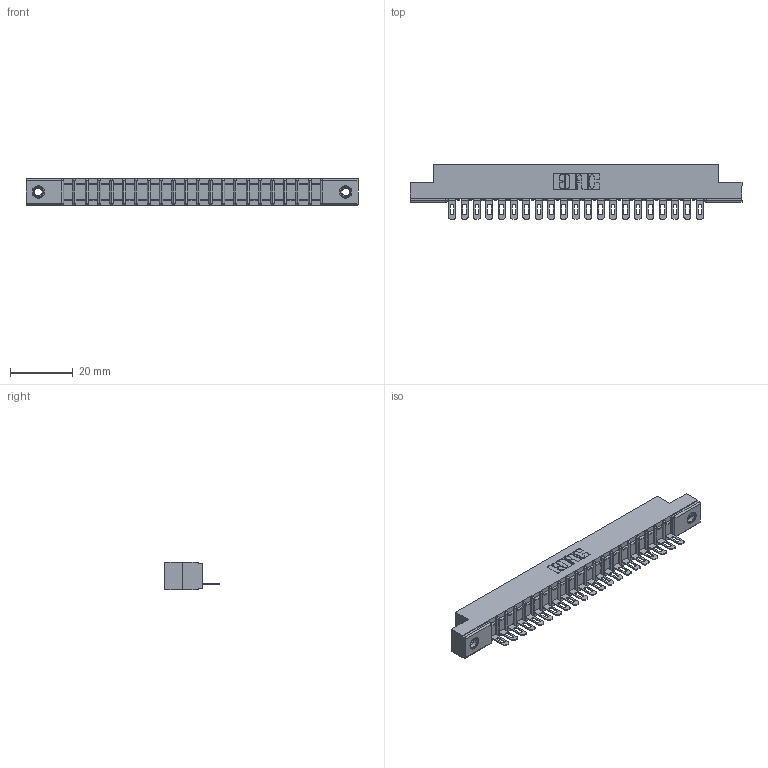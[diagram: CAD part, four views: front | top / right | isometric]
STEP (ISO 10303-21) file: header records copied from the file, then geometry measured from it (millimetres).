
FILE_DESCRIPTION (( 'STEP AP203' ), '1' );
FILE_NAME ('357-021-501-107.STEP', '2019-09-16T22:37:38', ( '' ), ( '' ), 'SwSTEP 2.0', 'SolidWorks 2016', '' );
FILE_SCHEMA (( 'CONFIG_CONTROL_DESIGN' ));
Length unit declared in the file: inch
Products named in the file (4): 345-250-001_345-250-005-103; 307-290-002_501; 307 Part_.156 Dia Mounting Holes; 357-021-501-107
Assembly tree (24 placements, depth 2):
  357-021-501-107
    307 Part_.156 Dia Mounting Holes
    307-290-002_501  x21
    345-250-001_345-250-005-103  x2
Bounding box: 106.22 x 17.42 x 8.71 mm (x, y, z)
Volume: 7016.9 mm3; surface area: 12883.8 mm2
Topology: 24 solids, 24 shells, 1796 faces, 5457 edges, 3570 vertices
Faces by surface type: plane 1026, cylinder 710, sphere 44, cone 12, torus 4
Entity records: 22571 total; most frequent: CARTESIAN_POINT 3783, ORIENTED_EDGE 3766, DIRECTION 3699, EDGE_CURVE 1883, VECTOR 1427, LINE 1427, VERTEX_POINT 1220, AXIS2_PLACEMENT_3D 1136
